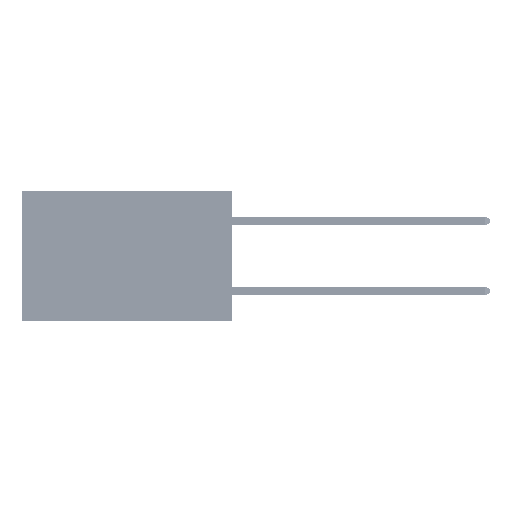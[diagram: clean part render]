
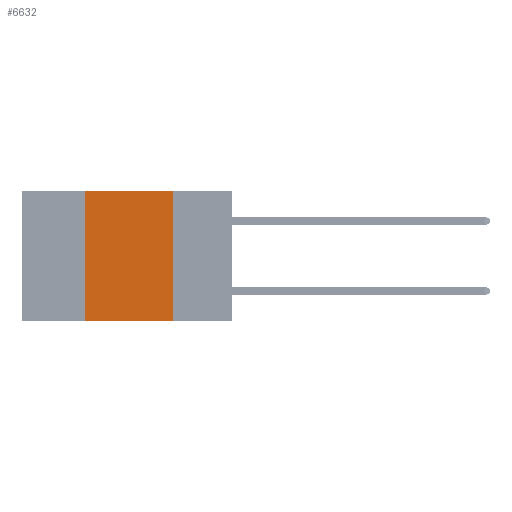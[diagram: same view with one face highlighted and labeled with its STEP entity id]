
A CAD part, left-side view. The second image highlights one B-rep face of the part: STEP entity #6632.
In plain terms, the highlighted planar face has unit normal (-1, 0, 0).
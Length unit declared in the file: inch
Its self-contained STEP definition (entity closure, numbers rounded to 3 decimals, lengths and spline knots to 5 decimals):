
#761 = CARTESIAN_POINT ( 'NONE',  ( 0., 0.17, -0.37 ) ) ;
#1945 = LINE ( 'NONE', #9104, #47723 ) ;
#4600 = ORIENTED_EDGE ( 'NONE', *, *, #26009, .F. ) ;
#6025 = VERTEX_POINT ( 'NONE', #761 ) ;
#6632 = ADVANCED_FACE ( 'NONE', ( #32283 ), #17780, .F. ) ;
#7080 = CARTESIAN_POINT ( 'NONE',  ( 0., 0.42, 0. ) ) ;
#8725 = ORIENTED_EDGE ( 'NONE', *, *, #10300, .T. ) ;
#9104 = CARTESIAN_POINT ( 'NONE',  ( 0., 0.17, 0. ) ) ;
#9776 = LINE ( 'NONE', #47836, #47934 ) ;
#10300 = EDGE_CURVE ( 'NONE', #11717, #6025, #9776, .T. ) ;
#11201 = LINE ( 'NONE', #22991, #42063 ) ;
#11717 = VERTEX_POINT ( 'NONE', #28690 ) ;
#14103 = DIRECTION ( 'NONE',  ( 1., 0., 0. ) ) ;
#17780 = PLANE ( 'NONE',  #27131 ) ;
#18763 = CARTESIAN_POINT ( 'NONE',  ( 0., 0.42, 0. ) ) ;
#18996 = LINE ( 'NONE', #18763, #20230 ) ;
#19279 = DIRECTION ( 'NONE',  ( 0., -1., 0. ) ) ;
#19555 = EDGE_CURVE ( 'NONE', #43899, #6025, #1945, .T. ) ;
#19722 = DIRECTION ( 'NONE',  ( 0., 0., 1. ) ) ;
#20230 = VECTOR ( 'NONE', #19722, 39.37008 ) ;
#22991 = CARTESIAN_POINT ( 'NONE',  ( 0., 0.6, 0. ) ) ;
#24070 = DIRECTION ( 'NONE',  ( 0., 0., -1. ) ) ;
#24487 = CARTESIAN_POINT ( 'NONE',  ( 0., 0.17, 0. ) ) ;
#25429 = VERTEX_POINT ( 'NONE', #7080 ) ;
#26009 = EDGE_CURVE ( 'NONE', #11717, #25429, #18996, .T. ) ;
#27131 = AXIS2_PLACEMENT_3D ( 'NONE', #47759, #14103, #29094 ) ;
#28690 = CARTESIAN_POINT ( 'NONE',  ( 0., 0.42, -0.37 ) ) ;
#28705 = EDGE_LOOP ( 'NONE', ( #46048, #42828, #4600, #8725 ) ) ;
#29094 = DIRECTION ( 'NONE',  ( 0., 0., -1. ) ) ;
#32283 = FACE_OUTER_BOUND ( 'NONE', #28705, .T. ) ;
#32596 = DIRECTION ( 'NONE',  ( 0., -1., 0. ) ) ;
#42063 = VECTOR ( 'NONE', #19279, 39.37008 ) ;
#42828 = ORIENTED_EDGE ( 'NONE', *, *, #42904, .F. ) ;
#42904 = EDGE_CURVE ( 'NONE', #25429, #43899, #11201, .T. ) ;
#43899 = VERTEX_POINT ( 'NONE', #24487 ) ;
#46048 = ORIENTED_EDGE ( 'NONE', *, *, #19555, .F. ) ;
#47723 = VECTOR ( 'NONE', #24070, 39.37008 ) ;
#47759 = CARTESIAN_POINT ( 'NONE',  ( 0., 0.6, 0. ) ) ;
#47836 = CARTESIAN_POINT ( 'NONE',  ( 0., 0.6, -0.37 ) ) ;
#47934 = VECTOR ( 'NONE', #32596, 39.37008 ) ;
